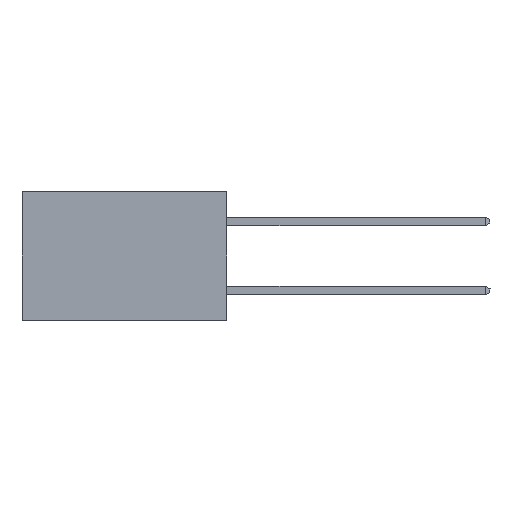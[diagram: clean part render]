
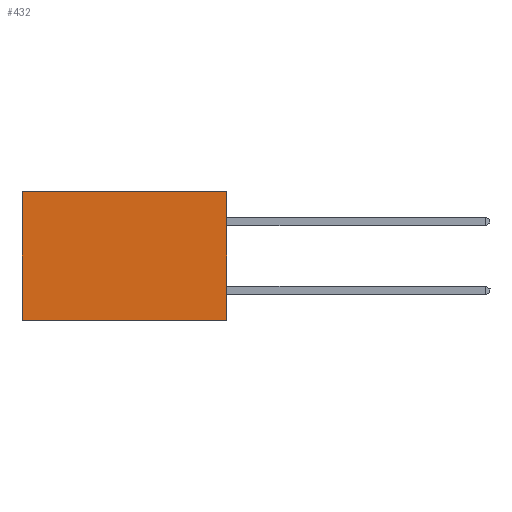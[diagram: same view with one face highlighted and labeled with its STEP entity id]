
A CAD part, left-side view. The second image highlights one B-rep face of the part: STEP entity #432.
In plain terms, the highlighted planar face has unit normal (-1, 0, 0).
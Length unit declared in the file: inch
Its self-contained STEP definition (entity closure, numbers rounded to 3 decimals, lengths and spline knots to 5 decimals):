
#36 = ORIENTED_EDGE ( 'NONE', *, *, #5451, .T. ) ;
#166 = ORIENTED_EDGE ( 'NONE', *, *, #3991, .F. ) ;
#210 = ORIENTED_EDGE ( 'NONE', *, *, #3689, .F. ) ;
#225 = ORIENTED_EDGE ( 'NONE', *, *, #2587, .T. ) ;
#413 = VECTOR ( 'NONE', #638, 39.37008 ) ;
#432 = ADVANCED_FACE ( 'NONE', ( #1196 ), #6448, .F. ) ;
#638 = DIRECTION ( 'NONE',  ( 0., 1., 0. ) ) ;
#657 = CARTESIAN_POINT ( 'NONE',  ( 0.277, 0., 0. ) ) ;
#797 = LINE ( 'NONE', #657, #3859 ) ;
#878 = CARTESIAN_POINT ( 'NONE',  ( 0.277, 0., -0.37 ) ) ;
#1196 = FACE_OUTER_BOUND ( 'NONE', #6884, .T. ) ;
#1248 = LINE ( 'NONE', #3049, #6918 ) ;
#1748 = DIRECTION ( 'NONE',  ( 0., 0., -1. ) ) ;
#2265 = CARTESIAN_POINT ( 'NONE',  ( 0.277, 0., 0. ) ) ;
#2310 = DIRECTION ( 'NONE',  ( 0., 0., -1. ) ) ;
#2415 = CARTESIAN_POINT ( 'NONE',  ( 0.277, 0.59, -0.37 ) ) ;
#2541 = VECTOR ( 'NONE', #1748, 39.37008 ) ;
#2587 = EDGE_CURVE ( 'NONE', #5559, #6042, #797, .T. ) ;
#2911 = DIRECTION ( 'NONE',  ( 0., 0., -1. ) ) ;
#3049 = CARTESIAN_POINT ( 'NONE',  ( 0.277, 0., -0.37 ) ) ;
#3290 = DIRECTION ( 'NONE',  ( 1., 0., 0. ) ) ;
#3689 = EDGE_CURVE ( 'NONE', #5559, #5158, #1248, .T. ) ;
#3859 = VECTOR ( 'NONE', #4215, 39.37008 ) ;
#3991 = EDGE_CURVE ( 'NONE', #5158, #4461, #6516, .T. ) ;
#4215 = DIRECTION ( 'NONE',  ( 0., 1., 0. ) ) ;
#4461 = VERTEX_POINT ( 'NONE', #6861 ) ;
#4813 = CARTESIAN_POINT ( 'NONE',  ( 0.277, 0.59, 0. ) ) ;
#5158 = VERTEX_POINT ( 'NONE', #7119 ) ;
#5451 = EDGE_CURVE ( 'NONE', #6042, #4461, #5483, .T. ) ;
#5483 = LINE ( 'NONE', #2415, #2541 ) ;
#5559 = VERTEX_POINT ( 'NONE', #2265 ) ;
#6042 = VERTEX_POINT ( 'NONE', #4813 ) ;
#6448 = PLANE ( 'NONE',  #7223 ) ;
#6516 = LINE ( 'NONE', #878, #413 ) ;
#6861 = CARTESIAN_POINT ( 'NONE',  ( 0.277, 0.59, -0.37 ) ) ;
#6884 = EDGE_LOOP ( 'NONE', ( #36, #166, #210, #225 ) ) ;
#6918 = VECTOR ( 'NONE', #2911, 39.37008 ) ;
#7047 = CARTESIAN_POINT ( 'NONE',  ( 0.277, 0., -0.37 ) ) ;
#7119 = CARTESIAN_POINT ( 'NONE',  ( 0.277, 0., -0.37 ) ) ;
#7223 = AXIS2_PLACEMENT_3D ( 'NONE', #7047, #3290, #2310 ) ;
